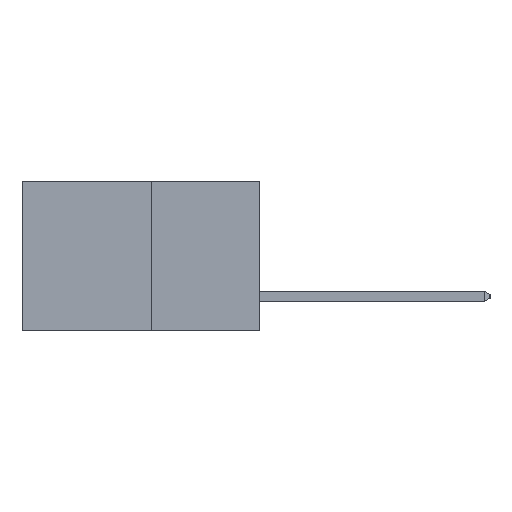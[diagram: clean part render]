
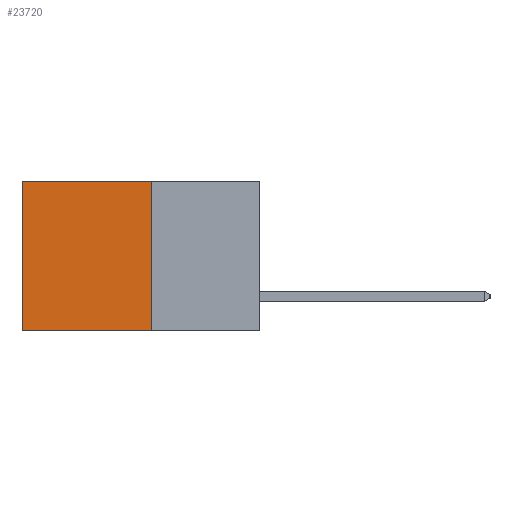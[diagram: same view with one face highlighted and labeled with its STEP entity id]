
A CAD part, left-side view. The second image highlights one B-rep face of the part: STEP entity #23720.
In plain terms, the highlighted planar face has unit normal (-1, 0, 0).
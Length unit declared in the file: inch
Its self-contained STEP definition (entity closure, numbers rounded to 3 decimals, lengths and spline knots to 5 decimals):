
#767 = ORIENTED_EDGE ( 'NONE', *, *, #3498, .F. ) ;
#1100 = VERTEX_POINT ( 'NONE', #2049 ) ;
#1377 = CARTESIAN_POINT ( 'NONE',  ( 0.277, 0.59, -0.37 ) ) ;
#1579 = DIRECTION ( 'NONE',  ( 0., 1., 0. ) ) ;
#2049 = CARTESIAN_POINT ( 'NONE',  ( 0.277, 0.27, 0. ) ) ;
#2796 = EDGE_CURVE ( 'NONE', #1100, #14334, #23912, .T. ) ;
#2941 = CARTESIAN_POINT ( 'NONE',  ( 0.277, 0.27, -0.37 ) ) ;
#3038 = ORIENTED_EDGE ( 'NONE', *, *, #2796, .T. ) ;
#3421 = DIRECTION ( 'NONE',  ( 0., 0., -1. ) ) ;
#3498 = EDGE_CURVE ( 'NONE', #5306, #5476, #4059, .T. ) ;
#3966 = LINE ( 'NONE', #1377, #13226 ) ;
#4059 = LINE ( 'NONE', #2941, #13306 ) ;
#5306 = VERTEX_POINT ( 'NONE', #14317 ) ;
#5455 = CARTESIAN_POINT ( 'NONE',  ( 0.277, 0.59, -0.37 ) ) ;
#5476 = VERTEX_POINT ( 'NONE', #5455 ) ;
#5632 = DIRECTION ( 'NONE',  ( 0., 0., -1. ) ) ;
#7006 = ORIENTED_EDGE ( 'NONE', *, *, #16032, .F. ) ;
#8025 = EDGE_LOOP ( 'NONE', ( #18356, #767, #7006, #3038 ) ) ;
#9340 = CARTESIAN_POINT ( 'NONE',  ( 0.277, 0.27, -0.37 ) ) ;
#9540 = PLANE ( 'NONE',  #18255 ) ;
#11288 = CARTESIAN_POINT ( 'NONE',  ( 0.277, 0.27, -0.37 ) ) ;
#11368 = DIRECTION ( 'NONE',  ( 0., 0., -1. ) ) ;
#12797 = VECTOR ( 'NONE', #5632, 39.37008 ) ;
#13226 = VECTOR ( 'NONE', #3421, 39.37008 ) ;
#13306 = VECTOR ( 'NONE', #1579, 39.37008 ) ;
#13633 = VECTOR ( 'NONE', #22048, 39.37008 ) ;
#13785 = CARTESIAN_POINT ( 'NONE',  ( 0.277, 0.27, 0. ) ) ;
#14317 = CARTESIAN_POINT ( 'NONE',  ( 0.277, 0.27, -0.37 ) ) ;
#14334 = VERTEX_POINT ( 'NONE', #17256 ) ;
#16032 = EDGE_CURVE ( 'NONE', #1100, #5306, #17670, .T. ) ;
#17256 = CARTESIAN_POINT ( 'NONE',  ( 0.277, 0.59, 0. ) ) ;
#17670 = LINE ( 'NONE', #9340, #12797 ) ;
#18255 = AXIS2_PLACEMENT_3D ( 'NONE', #11288, #22338, #11368 ) ;
#18356 = ORIENTED_EDGE ( 'NONE', *, *, #23547, .T. ) ;
#22048 = DIRECTION ( 'NONE',  ( 0., 1., 0. ) ) ;
#22338 = DIRECTION ( 'NONE',  ( 1., 0., 0. ) ) ;
#23222 = FACE_OUTER_BOUND ( 'NONE', #8025, .T. ) ;
#23547 = EDGE_CURVE ( 'NONE', #14334, #5476, #3966, .T. ) ;
#23720 = ADVANCED_FACE ( 'NONE', ( #23222 ), #9540, .F. ) ;
#23912 = LINE ( 'NONE', #13785, #13633 ) ;
